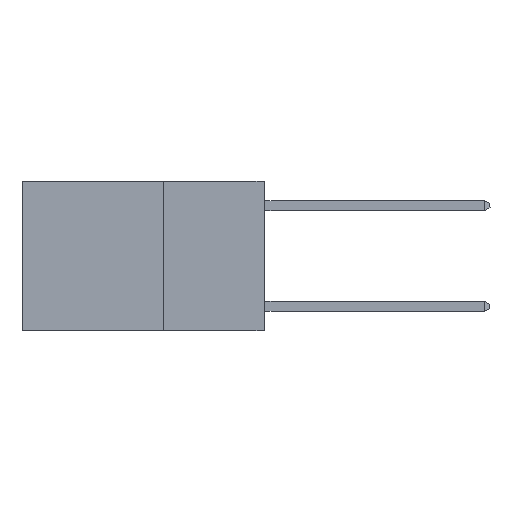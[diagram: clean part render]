
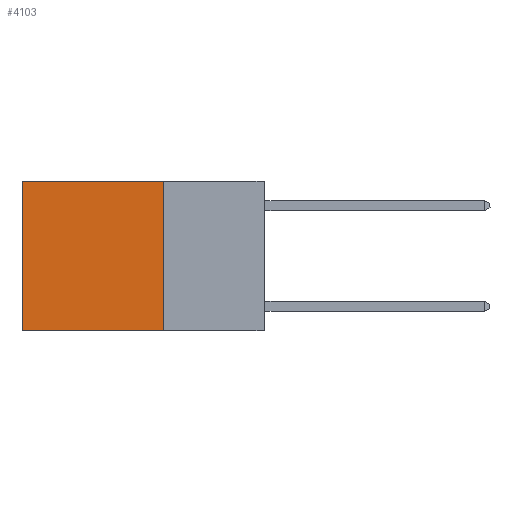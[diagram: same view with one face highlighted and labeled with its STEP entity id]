
A CAD part, left-side view. The second image highlights one B-rep face of the part: STEP entity #4103.
In plain terms, the highlighted planar face has unit normal (-1, 0, 0).
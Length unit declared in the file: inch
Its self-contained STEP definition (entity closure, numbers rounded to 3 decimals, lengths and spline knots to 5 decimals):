
#723 = DIRECTION ( 'NONE',  ( 0., 0., -1. ) ) ;
#1057 = PLANE ( 'NONE',  #2925 ) ;
#1189 = VECTOR ( 'NONE', #4243, 39.37008 ) ;
#1495 = EDGE_CURVE ( 'NONE', #4787, #4825, #10225, .T. ) ;
#1515 = DIRECTION ( 'NONE',  ( 1., 0., 0. ) ) ;
#2003 = VERTEX_POINT ( 'NONE', #6390 ) ;
#2099 = LINE ( 'NONE', #6671, #4319 ) ;
#2261 = EDGE_CURVE ( 'NONE', #2003, #5343, #9043, .T. ) ;
#2925 = AXIS2_PLACEMENT_3D ( 'NONE', #8797, #1515, #723 ) ;
#3577 = CARTESIAN_POINT ( 'NONE',  ( 0.2625, 0.6, 0. ) ) ;
#3935 = CARTESIAN_POINT ( 'NONE',  ( 0.2625, 0.6, -0.37 ) ) ;
#4029 = DIRECTION ( 'NONE',  ( 0., 1., 0. ) ) ;
#4103 = ADVANCED_FACE ( 'NONE', ( #6256 ), #1057, .F. ) ;
#4243 = DIRECTION ( 'NONE',  ( 0., 1., 0. ) ) ;
#4319 = VECTOR ( 'NONE', #11329, 39.37008 ) ;
#4787 = VERTEX_POINT ( 'NONE', #10899 ) ;
#4825 = VERTEX_POINT ( 'NONE', #3935 ) ;
#5036 = CARTESIAN_POINT ( 'NONE',  ( 0.2625, 0.25, 0. ) ) ;
#5104 = VECTOR ( 'NONE', #4029, 39.37008 ) ;
#5343 = VERTEX_POINT ( 'NONE', #3577 ) ;
#5822 = EDGE_CURVE ( 'NONE', #5343, #4825, #2099, .T. ) ;
#6037 = ORIENTED_EDGE ( 'NONE', *, *, #2261, .T. ) ;
#6171 = CARTESIAN_POINT ( 'NONE',  ( 0.2625, 0.25, -0.37 ) ) ;
#6256 = FACE_OUTER_BOUND ( 'NONE', #7706, .T. ) ;
#6281 = VECTOR ( 'NONE', #9244, 39.37008 ) ;
#6390 = CARTESIAN_POINT ( 'NONE',  ( 0.2625, 0.25, 0. ) ) ;
#6671 = CARTESIAN_POINT ( 'NONE',  ( 0.2625, 0.6, 0. ) ) ;
#6990 = ORIENTED_EDGE ( 'NONE', *, *, #10701, .F. ) ;
#7154 = LINE ( 'NONE', #11558, #6281 ) ;
#7706 = EDGE_LOOP ( 'NONE', ( #9059, #9213, #6990, #6037 ) ) ;
#8797 = CARTESIAN_POINT ( 'NONE',  ( 0.2625, 0.25, 0. ) ) ;
#9043 = LINE ( 'NONE', #5036, #5104 ) ;
#9059 = ORIENTED_EDGE ( 'NONE', *, *, #5822, .T. ) ;
#9213 = ORIENTED_EDGE ( 'NONE', *, *, #1495, .F. ) ;
#9244 = DIRECTION ( 'NONE',  ( 0., 0., -1. ) ) ;
#10225 = LINE ( 'NONE', #6171, #1189 ) ;
#10701 = EDGE_CURVE ( 'NONE', #2003, #4787, #7154, .T. ) ;
#10899 = CARTESIAN_POINT ( 'NONE',  ( 0.2625, 0.25, -0.37 ) ) ;
#11329 = DIRECTION ( 'NONE',  ( 0., 0., -1. ) ) ;
#11558 = CARTESIAN_POINT ( 'NONE',  ( 0.2625, 0.25, 0. ) ) ;
